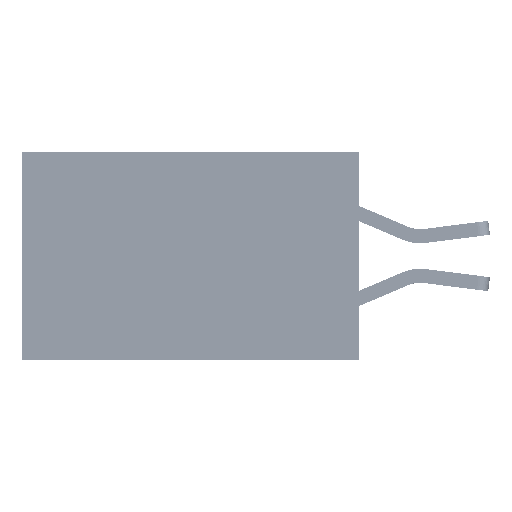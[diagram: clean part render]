
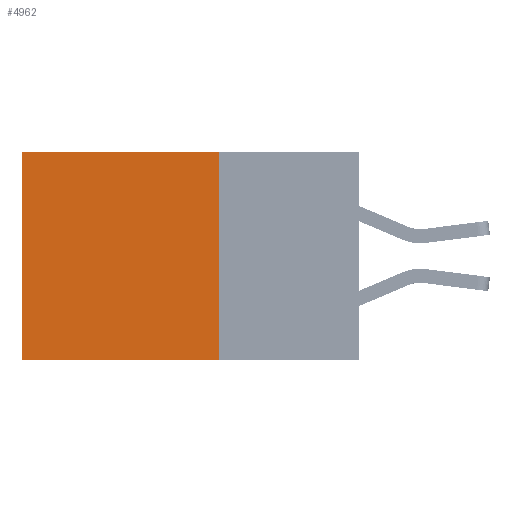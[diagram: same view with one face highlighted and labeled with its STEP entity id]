
A CAD part, left-side view. The second image highlights one B-rep face of the part: STEP entity #4962.
In plain terms, the highlighted planar face has unit normal (-1, 0, 0).
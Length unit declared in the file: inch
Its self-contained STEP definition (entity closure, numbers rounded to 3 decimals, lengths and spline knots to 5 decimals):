
#783 = VERTEX_POINT ( 'NONE', #24878 ) ;
#2567 = VERTEX_POINT ( 'NONE', #20098 ) ;
#3227 = CARTESIAN_POINT ( 'NONE',  ( 0.2875, 0.25, -0.37 ) ) ;
#4962 = ADVANCED_FACE ( 'NONE', ( #9908 ), #15189, .F. ) ;
#5133 = VERTEX_POINT ( 'NONE', #25530 ) ;
#9100 = CARTESIAN_POINT ( 'NONE',  ( 0.2875, 0.25, 0. ) ) ;
#9908 = FACE_OUTER_BOUND ( 'NONE', #36614, .T. ) ;
#10095 = ORIENTED_EDGE ( 'NONE', *, *, #39155, .F. ) ;
#15011 = CARTESIAN_POINT ( 'NONE',  ( 0.2875, 0.25, 0. ) ) ;
#15140 = DIRECTION ( 'NONE',  ( 0., 1., 0. ) ) ;
#15189 = PLANE ( 'NONE',  #38249 ) ;
#15705 = DIRECTION ( 'NONE',  ( 0., 1., 0. ) ) ;
#15968 = ORIENTED_EDGE ( 'NONE', *, *, #16477, .F. ) ;
#16477 = EDGE_CURVE ( 'NONE', #19320, #783, #19865, .T. ) ;
#18357 = VECTOR ( 'NONE', #35839, 39.37008 ) ;
#18564 = LINE ( 'NONE', #15011, #32020 ) ;
#19320 = VERTEX_POINT ( 'NONE', #20075 ) ;
#19865 = LINE ( 'NONE', #29505, #18357 ) ;
#20075 = CARTESIAN_POINT ( 'NONE',  ( 0.2875, 0.25, 0. ) ) ;
#20098 = CARTESIAN_POINT ( 'NONE',  ( 0.2875, 0.6, 0. ) ) ;
#20249 = EDGE_CURVE ( 'NONE', #19320, #2567, #18564, .T. ) ;
#20885 = DIRECTION ( 'NONE',  ( 0., 0., -1. ) ) ;
#22140 = VECTOR ( 'NONE', #15705, 39.37008 ) ;
#24878 = CARTESIAN_POINT ( 'NONE',  ( 0.2875, 0.25, -0.37 ) ) ;
#25530 = CARTESIAN_POINT ( 'NONE',  ( 0.2875, 0.6, -0.37 ) ) ;
#29204 = LINE ( 'NONE', #3227, #22140 ) ;
#29505 = CARTESIAN_POINT ( 'NONE',  ( 0.2875, 0.25, 0. ) ) ;
#29563 = VECTOR ( 'NONE', #20885, 39.37008 ) ;
#30931 = DIRECTION ( 'NONE',  ( 0., 0., -1. ) ) ;
#32020 = VECTOR ( 'NONE', #15140, 39.37008 ) ;
#33508 = LINE ( 'NONE', #34063, #29563 ) ;
#34063 = CARTESIAN_POINT ( 'NONE',  ( 0.2875, 0.6, 0. ) ) ;
#34715 = EDGE_CURVE ( 'NONE', #2567, #5133, #33508, .T. ) ;
#35839 = DIRECTION ( 'NONE',  ( 0., 0., -1. ) ) ;
#36549 = ORIENTED_EDGE ( 'NONE', *, *, #20249, .T. ) ;
#36614 = EDGE_LOOP ( 'NONE', ( #40241, #10095, #15968, #36549 ) ) ;
#37668 = DIRECTION ( 'NONE',  ( 1., 0., 0. ) ) ;
#38249 = AXIS2_PLACEMENT_3D ( 'NONE', #9100, #37668, #30931 ) ;
#39155 = EDGE_CURVE ( 'NONE', #783, #5133, #29204, .T. ) ;
#40241 = ORIENTED_EDGE ( 'NONE', *, *, #34715, .T. ) ;
